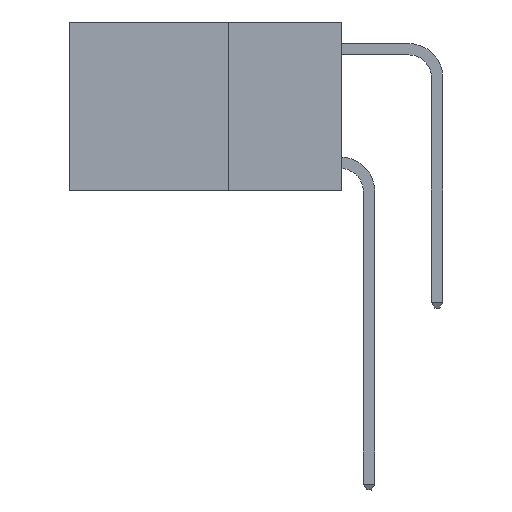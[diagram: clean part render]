
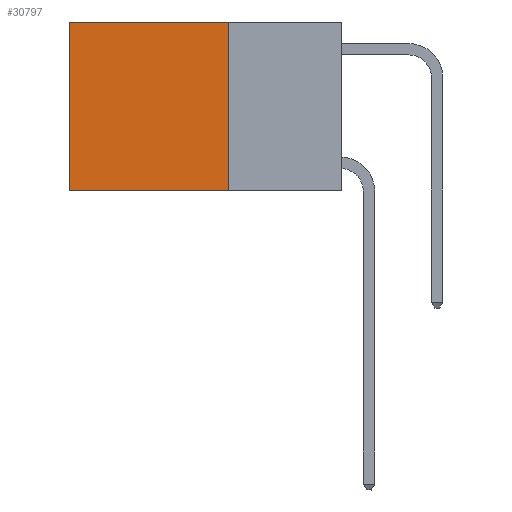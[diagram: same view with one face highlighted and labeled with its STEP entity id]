
A CAD part, left-side view. The second image highlights one B-rep face of the part: STEP entity #30797.
In plain terms, the highlighted planar face has unit normal (-1, 0, 0).
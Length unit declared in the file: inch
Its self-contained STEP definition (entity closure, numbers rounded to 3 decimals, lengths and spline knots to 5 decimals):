
#314 = FACE_OUTER_BOUND ( 'NONE', #3706, .T. ) ;
#1399 = CARTESIAN_POINT ( 'NONE',  ( 0.2625, 0.25, 0. ) ) ;
#1491 = LINE ( 'NONE', #30994, #21990 ) ;
#3706 = EDGE_LOOP ( 'NONE', ( #18024, #22140, #29506, #21145 ) ) ;
#3784 = VERTEX_POINT ( 'NONE', #7953 ) ;
#4341 = VERTEX_POINT ( 'NONE', #24531 ) ;
#4382 = VECTOR ( 'NONE', #24753, 39.37008 ) ;
#4503 = DIRECTION ( 'NONE',  ( 0., 1., 0. ) ) ;
#4807 = LINE ( 'NONE', #8932, #4382 ) ;
#5720 = LINE ( 'NONE', #23284, #29513 ) ;
#5796 = EDGE_CURVE ( 'NONE', #3784, #23498, #1491, .T. ) ;
#7953 = CARTESIAN_POINT ( 'NONE',  ( 0.2625, 0.25, -0.37 ) ) ;
#8232 = PLANE ( 'NONE',  #8784 ) ;
#8784 = AXIS2_PLACEMENT_3D ( 'NONE', #1399, #19771, #12010 ) ;
#8932 = CARTESIAN_POINT ( 'NONE',  ( 0.2625, 0.6, 0. ) ) ;
#12010 = DIRECTION ( 'NONE',  ( 0., 0., -1. ) ) ;
#12314 = LINE ( 'NONE', #19842, #20823 ) ;
#18024 = ORIENTED_EDGE ( 'NONE', *, *, #26268, .T. ) ;
#19771 = DIRECTION ( 'NONE',  ( 1., 0., 0. ) ) ;
#19842 = CARTESIAN_POINT ( 'NONE',  ( 0.2625, 0.25, 0. ) ) ;
#20823 = VECTOR ( 'NONE', #23434, 39.37008 ) ;
#21145 = ORIENTED_EDGE ( 'NONE', *, *, #29574, .T. ) ;
#21990 = VECTOR ( 'NONE', #4503, 39.37008 ) ;
#22140 = ORIENTED_EDGE ( 'NONE', *, *, #5796, .F. ) ;
#23284 = CARTESIAN_POINT ( 'NONE',  ( 0.2625, 0.25, 0. ) ) ;
#23434 = DIRECTION ( 'NONE',  ( 0., 1., 0. ) ) ;
#23498 = VERTEX_POINT ( 'NONE', #28080 ) ;
#23508 = DIRECTION ( 'NONE',  ( 0., 0., -1. ) ) ;
#24531 = CARTESIAN_POINT ( 'NONE',  ( 0.2625, 0.25, 0. ) ) ;
#24753 = DIRECTION ( 'NONE',  ( 0., 0., -1. ) ) ;
#25962 = CARTESIAN_POINT ( 'NONE',  ( 0.2625, 0.6, 0. ) ) ;
#26268 = EDGE_CURVE ( 'NONE', #34077, #23498, #4807, .T. ) ;
#28080 = CARTESIAN_POINT ( 'NONE',  ( 0.2625, 0.6, -0.37 ) ) ;
#29506 = ORIENTED_EDGE ( 'NONE', *, *, #32209, .F. ) ;
#29513 = VECTOR ( 'NONE', #23508, 39.37008 ) ;
#29574 = EDGE_CURVE ( 'NONE', #4341, #34077, #12314, .T. ) ;
#30797 = ADVANCED_FACE ( 'NONE', ( #314 ), #8232, .F. ) ;
#30994 = CARTESIAN_POINT ( 'NONE',  ( 0.2625, 0.25, -0.37 ) ) ;
#32209 = EDGE_CURVE ( 'NONE', #4341, #3784, #5720, .T. ) ;
#34077 = VERTEX_POINT ( 'NONE', #25962 ) ;
